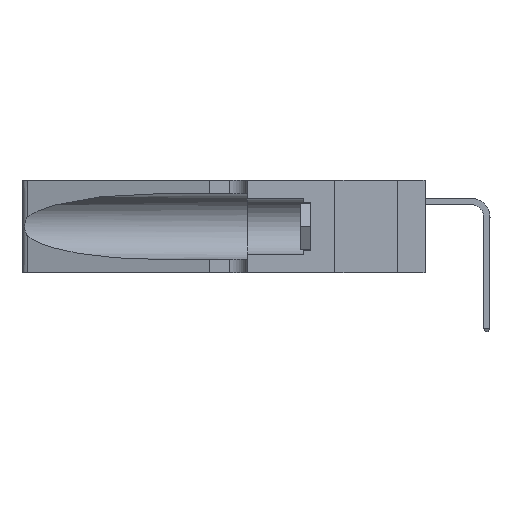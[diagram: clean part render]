
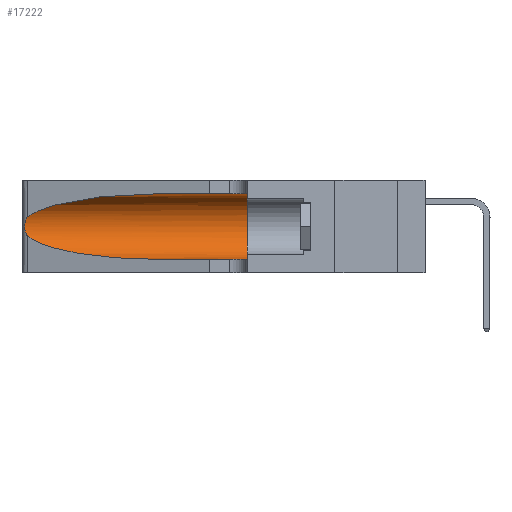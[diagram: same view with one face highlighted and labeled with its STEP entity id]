
A CAD part, left-side view. The second image highlights one B-rep face of the part: STEP entity #17222.
In plain terms, the highlighted cylindrical face has radius 3.308 mm (diameter 6.617 mm), a partial arc.
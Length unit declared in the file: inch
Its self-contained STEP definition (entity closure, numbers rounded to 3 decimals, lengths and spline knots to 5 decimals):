
#328 = CARTESIAN_POINT ( 'NONE',  ( 0.18966, 0.96281, 0.05475 ) ) ;
#421 = FACE_OUTER_BOUND ( 'NONE', #11784, .T. ) ;
#1415 = CARTESIAN_POINT ( 'NONE',  ( 0.1305, 0.72297, 0.05475 ) ) ;
#2178 = CARTESIAN_POINT ( 'NONE',  ( 0.26017, 1.23833, 0.17102 ) ) ;
#3368 = DIRECTION ( 'NONE',  ( 0., 0., -1. ) ) ;
#3817 = VERTEX_POINT ( 'NONE', #18692 ) ;
#4899 = DIRECTION ( 'NONE',  ( 0., -1., 0. ) ) ;
#5101 = CARTESIAN_POINT ( 'NONE',  ( 0.25789, 1.23486, 0.15765 ) ) ;
#5395 = EDGE_CURVE ( 'NONE', #31065, #31700, #29569, .T. ) ;
#6547 = ORIENTED_EDGE ( 'NONE', *, *, #23146, .F. ) ;
#7091 = VECTOR ( 'NONE', #4899, 39.37008 ) ;
#7835 = CARTESIAN_POINT ( 'NONE',  ( 0.25487, 1.22718, 0.22369 ) ) ;
#7954 = CARTESIAN_POINT ( 'NONE',  ( 0.25555, 1.22993, 0.14849 ) ) ;
#7978 = EDGE_CURVE ( 'NONE', #31700, #29466, #13682, .T. ) ;
#8166 = ORIENTED_EDGE ( 'NONE', *, *, #11146, .T. ) ;
#8737 = B_SPLINE_CURVE_WITH_KNOTS ( 'NONE', 3,
 ( #7835, #24698, #30307, #13483, #33106, #16284, #35858, #19126, #2178, #21979, #5101, #24829, #7954, #27597 ),
 .UNSPECIFIED., .F., .F.,
 ( 4, 2, 2, 2, 2, 2, 4 ),
 ( 0., 0.00027, 0.00053, 0.00107, 0.0016, 0.00187, 0.00214 ),
 .UNSPECIFIED. ) ;
#9619 = CARTESIAN_POINT ( 'NONE',  ( 0.1305, 0.35, 0.185 ) ) ;
#10465 = VECTOR ( 'NONE', #15841, 39.37008 ) ;
#10812 = CARTESIAN_POINT ( 'NONE',  ( 0.18966, 0.96281, 0.31525 ) ) ;
#11146 = EDGE_CURVE ( 'NONE', #31481, #30001, #16022, .T. ) ;
#11784 = EDGE_LOOP ( 'NONE', ( #8166, #28207, #29132, #16322, #24996, #6547 ) ) ;
#12439 = DIRECTION ( 'NONE',  ( 0., 0., 1. ) ) ;
#13483 = CARTESIAN_POINT ( 'NONE',  ( 0.25787, 1.23484, 0.2124 ) ) ;
#13520 = EDGE_CURVE ( 'NONE', #3817, #29466, #26383, .T. ) ;
#13654 = CARTESIAN_POINT ( 'NONE',  ( 0.1305, 0.72297, 0.31525 ) ) ;
#13682 = LINE ( 'NONE', #16102, #7091 ) ;
#14464 = AXIS2_PLACEMENT_3D ( 'NONE', #9619, #29252, #12439 ) ;
#15841 = DIRECTION ( 'NONE',  ( 0., -1., 0. ) ) ;
#16022 =( BOUNDED_CURVE ( )  B_SPLINE_CURVE ( 3, ( #13654, #10812, #19168, #33257 ),
 .UNSPECIFIED., .F., .F. ) 
 B_SPLINE_CURVE_WITH_KNOTS ( ( 4, 4 ),
 ( 1.5708, 2.84003 ),
 .UNSPECIFIED. ) 
 CURVE ( )  GEOMETRIC_REPRESENTATION_ITEM ( )  RATIONAL_B_SPLINE_CURVE ( ( 1., 0.87, 0.87, 1. ) ) 
 REPRESENTATION_ITEM ( '' )  );
#16102 = CARTESIAN_POINT ( 'NONE',  ( 0.1305, 1.61858, 0.05475 ) ) ;
#16284 = CARTESIAN_POINT ( 'NONE',  ( 0.26018, 1.23835, 0.19895 ) ) ;
#16322 = ORIENTED_EDGE ( 'NONE', *, *, #7978, .T. ) ;
#17222 = ADVANCED_FACE ( 'NONE', ( #421 ), #36051, .F. ) ;
#17294 = CARTESIAN_POINT ( 'NONE',  ( 0.25487, 1.22718, 0.14631 ) ) ;
#18692 = CARTESIAN_POINT ( 'NONE',  ( 0.1305, 0.35, 0.31525 ) ) ;
#19126 = CARTESIAN_POINT ( 'NONE',  ( 0.26075, 1.23896, 0.178 ) ) ;
#19168 = CARTESIAN_POINT ( 'NONE',  ( 0.2373, 1.15595, 0.28018 ) ) ;
#20137 = CARTESIAN_POINT ( 'NONE',  ( 0.1305, 0.72297, 0.05475 ) ) ;
#20295 = DIRECTION ( 'NONE',  ( 0., -1., 0. ) ) ;
#21863 = CARTESIAN_POINT ( 'NONE',  ( 0.25487, 1.22718, 0.22369 ) ) ;
#21979 = CARTESIAN_POINT ( 'NONE',  ( 0.25856, 1.23593, 0.16098 ) ) ;
#23092 = CARTESIAN_POINT ( 'NONE',  ( 0.1305, 0.72297, 0.31525 ) ) ;
#23146 = EDGE_CURVE ( 'NONE', #31481, #3817, #32861, .T. ) ;
#24468 = AXIS2_PLACEMENT_3D ( 'NONE', #34246, #20295, #3368 ) ;
#24698 = CARTESIAN_POINT ( 'NONE',  ( 0.25555, 1.22994, 0.2215 ) ) ;
#24829 = CARTESIAN_POINT ( 'NONE',  ( 0.25639, 1.23186, 0.15144 ) ) ;
#24996 = ORIENTED_EDGE ( 'NONE', *, *, #13520, .F. ) ;
#26383 = CIRCLE ( 'NONE', #14464, 0.13025 ) ;
#27597 = CARTESIAN_POINT ( 'NONE',  ( 0.25487, 1.22718, 0.14631 ) ) ;
#28207 = ORIENTED_EDGE ( 'NONE', *, *, #31208, .T. ) ;
#29132 = ORIENTED_EDGE ( 'NONE', *, *, #5395, .T. ) ;
#29252 = DIRECTION ( 'NONE',  ( 0., 1., 0. ) ) ;
#29466 = VERTEX_POINT ( 'NONE', #33122 ) ;
#29569 =( BOUNDED_CURVE ( )  B_SPLINE_CURVE ( 3, ( #17294, #34085, #328, #20137 ),
 .UNSPECIFIED., .F., .F. ) 
 B_SPLINE_CURVE_WITH_KNOTS ( ( 4, 4 ),
 ( 3.44316, 4.71239 ),
 .UNSPECIFIED. ) 
 CURVE ( )  GEOMETRIC_REPRESENTATION_ITEM ( )  RATIONAL_B_SPLINE_CURVE ( ( 1., 0.87, 0.87, 1. ) ) 
 REPRESENTATION_ITEM ( '' )  );
#29708 = CARTESIAN_POINT ( 'NONE',  ( 0.25487, 1.22718, 0.14631 ) ) ;
#30001 = VERTEX_POINT ( 'NONE', #21863 ) ;
#30307 = CARTESIAN_POINT ( 'NONE',  ( 0.25639, 1.23184, 0.21858 ) ) ;
#31065 = VERTEX_POINT ( 'NONE', #29708 ) ;
#31208 = EDGE_CURVE ( 'NONE', #30001, #31065, #8737, .T. ) ;
#31481 = VERTEX_POINT ( 'NONE', #23092 ) ;
#31700 = VERTEX_POINT ( 'NONE', #1415 ) ;
#32861 = LINE ( 'NONE', #35430, #10465 ) ;
#33106 = CARTESIAN_POINT ( 'NONE',  ( 0.25854, 1.2359, 0.20912 ) ) ;
#33122 = CARTESIAN_POINT ( 'NONE',  ( 0.1305, 0.35, 0.05475 ) ) ;
#33257 = CARTESIAN_POINT ( 'NONE',  ( 0.25487, 1.22718, 0.22369 ) ) ;
#34085 = CARTESIAN_POINT ( 'NONE',  ( 0.2373, 1.15595, 0.08982 ) ) ;
#34246 = CARTESIAN_POINT ( 'NONE',  ( 0.1305, 1.61858, 0.185 ) ) ;
#35430 = CARTESIAN_POINT ( 'NONE',  ( 0.1305, 1.61858, 0.31525 ) ) ;
#35858 = CARTESIAN_POINT ( 'NONE',  ( 0.26075, 1.23896, 0.19203 ) ) ;
#36051 = CYLINDRICAL_SURFACE ( 'NONE', #24468, 0.13025 ) ;
